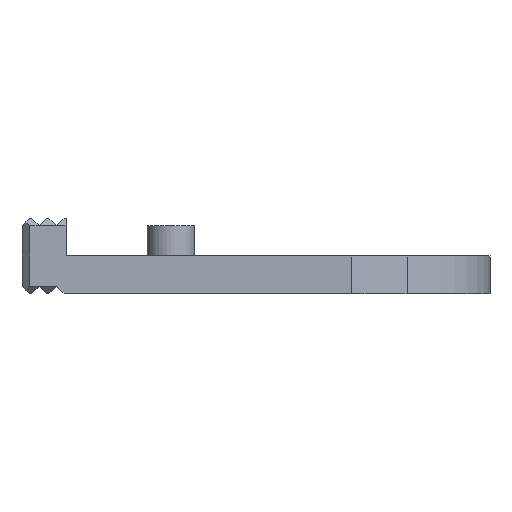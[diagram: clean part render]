
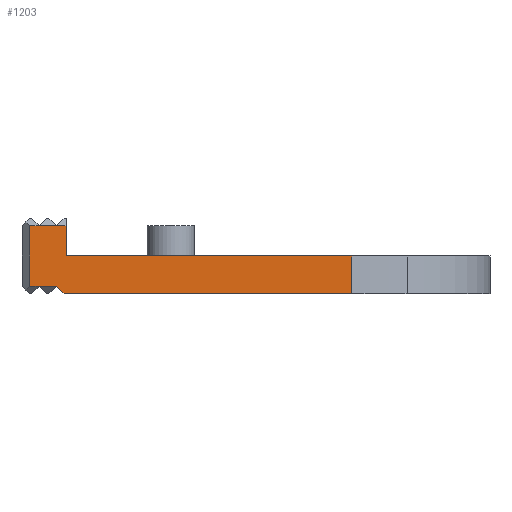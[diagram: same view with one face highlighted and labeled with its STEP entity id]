
A CAD part, left-side view. The second image highlights one B-rep face of the part: STEP entity #1203.
In plain terms, the highlighted planar face has unit normal (-1, 0, 0).
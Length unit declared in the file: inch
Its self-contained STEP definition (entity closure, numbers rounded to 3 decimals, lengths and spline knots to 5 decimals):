
#55=PLANE('',#1316);
#107=FACE_OUTER_BOUND('',#179,.T.);
#179=EDGE_LOOP('',(#970,#971,#972,#973,#974,#975,#976,#977,#978,#979,#980));
#274=LINE('',#1755,#415);
#289=LINE('',#1812,#430);
#294=LINE('',#1831,#435);
#328=LINE('',#1917,#469);
#332=LINE('',#1924,#473);
#334=LINE('',#1928,#475);
#335=LINE('',#1930,#476);
#336=LINE('',#1932,#477);
#337=LINE('',#1934,#478);
#338=LINE('',#1935,#479);
#339=LINE('',#1936,#480);
#415=VECTOR('',#1402,0.93952);
#430=VECTOR('',#1449,0.1);
#435=VECTOR('',#1464,0.94619);
#469=VECTOR('',#1536,0.03536);
#473=VECTOR('',#1544,0.3937);
#475=VECTOR('',#1548,0.3937);
#476=VECTOR('',#1549,0.3937);
#477=VECTOR('',#1550,0.3937);
#478=VECTOR('',#1551,0.3937);
#479=VECTOR('',#1552,0.3937);
#480=VECTOR('',#1553,0.125);
#557=VERTEX_POINT('',#1752);
#558=VERTEX_POINT('',#1754);
#584=VERTEX_POINT('',#1810);
#592=VERTEX_POINT('',#1828);
#593=VERTEX_POINT('',#1830);
#617=VERTEX_POINT('',#1888);
#626=VERTEX_POINT('',#1916);
#628=VERTEX_POINT('',#1927);
#629=VERTEX_POINT('',#1929);
#630=VERTEX_POINT('',#1931);
#631=VERTEX_POINT('',#1933);
#673=EDGE_CURVE('',#558,#557,#274,.T.);
#702=EDGE_CURVE('',#557,#584,#289,.T.);
#711=EDGE_CURVE('',#592,#593,#294,.T.);
#754=EDGE_CURVE('',#626,#593,#328,.T.);
#758=EDGE_CURVE('',#626,#617,#332,.T.);
#760=EDGE_CURVE('',#628,#584,#334,.T.);
#761=EDGE_CURVE('',#629,#628,#335,.T.);
#762=EDGE_CURVE('',#630,#629,#336,.T.);
#763=EDGE_CURVE('',#631,#630,#337,.T.);
#764=EDGE_CURVE('',#617,#631,#338,.T.);
#765=EDGE_CURVE('',#558,#592,#339,.T.);
#970=ORIENTED_EDGE('',*,*,#673,.T.);
#971=ORIENTED_EDGE('',*,*,#702,.T.);
#972=ORIENTED_EDGE('',*,*,#760,.F.);
#973=ORIENTED_EDGE('',*,*,#761,.F.);
#974=ORIENTED_EDGE('',*,*,#762,.F.);
#975=ORIENTED_EDGE('',*,*,#763,.F.);
#976=ORIENTED_EDGE('',*,*,#764,.F.);
#977=ORIENTED_EDGE('',*,*,#758,.F.);
#978=ORIENTED_EDGE('',*,*,#754,.T.);
#979=ORIENTED_EDGE('',*,*,#711,.F.);
#980=ORIENTED_EDGE('',*,*,#765,.F.);
#1203=ADVANCED_FACE('',(#107),#55,.T.);
#1316=AXIS2_PLACEMENT_3D('',#1926,#1546,#1547);
#1402=DIRECTION('',(0.,1.,0.));
#1449=DIRECTION('',(0.,0.,1.));
#1464=DIRECTION('',(0.,1.,0.));
#1536=DIRECTION('',(0.,-0.707,-0.707));
#1544=DIRECTION('',(0.,1.,0.));
#1546=DIRECTION('center_axis',(-1.,0.,0.));
#1547=DIRECTION('ref_axis',(0.,0.,1.));
#1548=DIRECTION('',(0.,-1.,0.));
#1549=DIRECTION('',(0.,-1.,0.));
#1550=DIRECTION('',(0.,-1.,0.));
#1551=DIRECTION('',(0.,0.,1.));
#1552=DIRECTION('',(0.,1.,0.));
#1553=DIRECTION('',(0.,0.,-1.));
#1752=CARTESIAN_POINT('',(-0.21256,1.33633,0.125));
#1754=CARTESIAN_POINT('',(-0.21256,0.39681,0.125));
#1755=CARTESIAN_POINT('',(-0.21256,0.39681,0.125));
#1810=CARTESIAN_POINT('',(-0.21256,1.33633,0.225));
#1812=CARTESIAN_POINT('',(-0.21256,1.33633,0.125));
#1828=CARTESIAN_POINT('',(-0.21256,0.39681,0.));
#1830=CARTESIAN_POINT('',(-0.21256,1.343,0.));
#1831=CARTESIAN_POINT('',(-0.21256,0.39681,0.));
#1888=CARTESIAN_POINT('',(-0.21256,1.42467,0.025));
#1916=CARTESIAN_POINT('',(-0.21256,1.368,0.025));
#1917=CARTESIAN_POINT('',(-0.21256,1.368,0.025));
#1924=CARTESIAN_POINT('',(-0.21256,1.23681,0.025));
#1926=CARTESIAN_POINT('Origin',(-0.21256,1.48133,0.25));
#1927=CARTESIAN_POINT('',(-0.21256,1.368,0.225));
#1928=CARTESIAN_POINT('',(-0.21256,1.23681,0.225));
#1929=CARTESIAN_POINT('',(-0.21256,1.42467,0.225));
#1930=CARTESIAN_POINT('',(-0.21256,1.23681,0.225));
#1931=CARTESIAN_POINT('',(-0.21256,1.45633,0.225));
#1932=CARTESIAN_POINT('',(-0.21256,1.23681,0.225));
#1933=CARTESIAN_POINT('',(-0.21256,1.45633,0.025));
#1934=CARTESIAN_POINT('',(-0.21256,1.45633,0.25));
#1935=CARTESIAN_POINT('',(-0.21256,1.23681,0.025));
#1936=CARTESIAN_POINT('',(-0.21256,0.39681,0.125));
